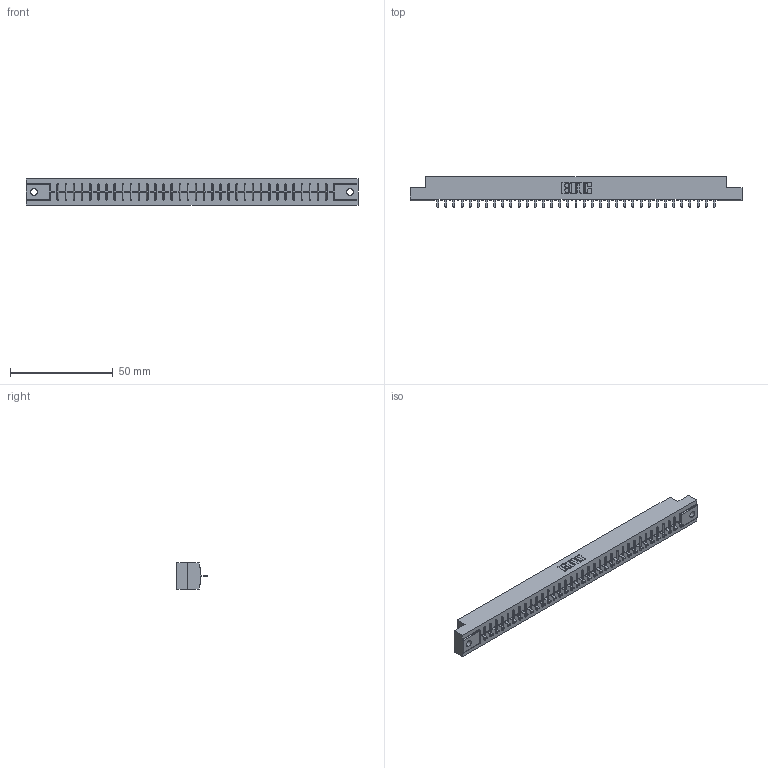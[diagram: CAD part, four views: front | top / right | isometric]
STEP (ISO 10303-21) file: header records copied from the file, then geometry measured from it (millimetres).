
FILE_DESCRIPTION (( 'STEP AP203' ), '1' );
FILE_NAME ('316-035-521-102.STEP', '2018-07-31T04:19:21', ( '' ), ( '' ), 'SwSTEP 2.0', 'SolidWorks 2016', '' );
FILE_SCHEMA (( 'CONFIG_CONTROL_DESIGN' ));
Length unit declared in the file: inch
Products named in the file (3): 316-035-521-102; 306 Part_.128 Dia; 306-290-001_121
Assembly tree (36 placements, depth 2):
  316-035-521-102
    306 Part_.128 Dia
    306-290-001_121  x35
Bounding box: 161.7 x 14.88 x 12.7 mm (x, y, z)
Volume: 17742.6 mm3; surface area: 17592.5 mm2
Topology: 36 solids, 36 shells, 2566 faces, 7211 edges, 4618 vertices
Faces by surface type: plane 1713, cylinder 713, sphere 140
Entity records: 33504 total; most frequent: CARTESIAN_POINT 5624, ORIENTED_EDGE 5574, DIRECTION 5547, EDGE_CURVE 2787, LINE 2177, VECTOR 2177, VERTEX_POINT 1762, AXIS2_PLACEMENT_3D 1685
